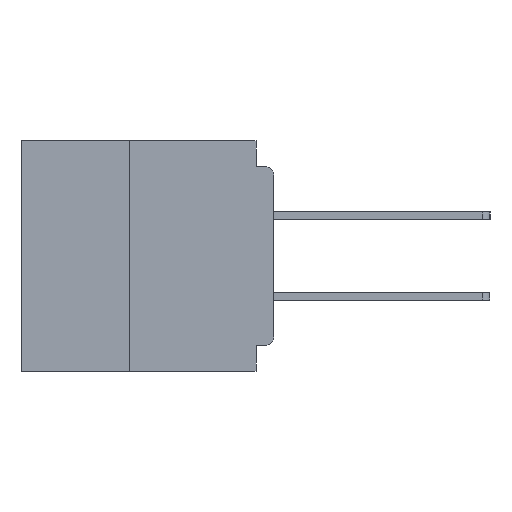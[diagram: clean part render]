
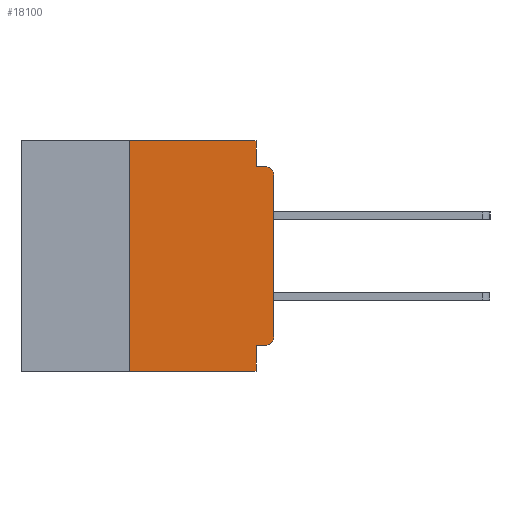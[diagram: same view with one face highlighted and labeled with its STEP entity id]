
A CAD part, left-side view. The second image highlights one B-rep face of the part: STEP entity #18100.
In plain terms, the highlighted planar face has unit normal (-1, 0, 0).
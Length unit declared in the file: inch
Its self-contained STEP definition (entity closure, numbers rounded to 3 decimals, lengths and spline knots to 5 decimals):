
#361 = VECTOR ( 'NONE', #4038, 39.37008 ) ;
#411 = CARTESIAN_POINT ( 'NONE',  ( 0., 0.031, -0.4 ) ) ;
#1312 = LINE ( 'NONE', #27914, #361 ) ;
#1744 = DIRECTION ( 'NONE',  ( 0., 0., -1. ) ) ;
#2793 = ORIENTED_EDGE ( 'NONE', *, *, #10416, .F. ) ;
#3578 = ORIENTED_EDGE ( 'NONE', *, *, #20698, .F. ) ;
#4038 = DIRECTION ( 'NONE',  ( 0., -1., 0. ) ) ;
#4580 = DIRECTION ( 'NONE',  ( 0., 1., 0. ) ) ;
#4935 = VECTOR ( 'NONE', #12124, 39.37008 ) ;
#5967 = VERTEX_POINT ( 'NONE', #23210 ) ;
#5987 = EDGE_CURVE ( 'NONE', #5967, #30522, #28568, .T. ) ;
#6387 = DIRECTION ( 'NONE',  ( 0., 0., -1. ) ) ;
#6660 = VECTOR ( 'NONE', #13336, 39.37008 ) ;
#6717 = EDGE_CURVE ( 'NONE', #25941, #8193, #11268, .T. ) ;
#6762 = VERTEX_POINT ( 'NONE', #13317 ) ;
#7190 = ORIENTED_EDGE ( 'NONE', *, *, #8110, .F. ) ;
#7269 = ORIENTED_EDGE ( 'NONE', *, *, #6717, .F. ) ;
#7526 = CIRCLE ( 'NONE', #22217, 0.015 ) ;
#7568 = LINE ( 'NONE', #28177, #6660 ) ;
#7718 = DIRECTION ( 'NONE',  ( -1., 0., 0. ) ) ;
#7893 = ORIENTED_EDGE ( 'NONE', *, *, #26180, .T. ) ;
#8110 = EDGE_CURVE ( 'NONE', #6762, #12100, #1312, .T. ) ;
#8193 = VERTEX_POINT ( 'NONE', #13462 ) ;
#8603 = EDGE_CURVE ( 'NONE', #12100, #25941, #36932, .T. ) ;
#9294 = FACE_OUTER_BOUND ( 'NONE', #30058, .T. ) ;
#10416 = EDGE_CURVE ( 'NONE', #21054, #30927, #36407, .T. ) ;
#10560 = CARTESIAN_POINT ( 'NONE',  ( 0., 0., -0.355 ) ) ;
#11268 = LINE ( 'NONE', #21096, #18243 ) ;
#11786 = VECTOR ( 'NONE', #23440, 39.37008 ) ;
#11883 = LINE ( 'NONE', #10560, #18884 ) ;
#12100 = VERTEX_POINT ( 'NONE', #33502 ) ;
#12124 = DIRECTION ( 'NONE',  ( 0., 0., -1. ) ) ;
#12818 = VECTOR ( 'NONE', #34408, 39.37008 ) ;
#13317 = CARTESIAN_POINT ( 'NONE',  ( 0., 0.25, 0. ) ) ;
#13336 = DIRECTION ( 'NONE',  ( 0., -1., 0. ) ) ;
#13462 = CARTESIAN_POINT ( 'NONE',  ( 0., 0.015, -0.045 ) ) ;
#13906 = DIRECTION ( 'NONE',  ( -1., 0., 0. ) ) ;
#14189 = DIRECTION ( 'NONE',  ( 0., -1., 0. ) ) ;
#15137 = CARTESIAN_POINT ( 'NONE',  ( 0., 0.031, -0.4 ) ) ;
#16322 = EDGE_CURVE ( 'NONE', #33196, #5967, #7526, .T. ) ;
#17006 = AXIS2_PLACEMENT_3D ( 'NONE', #37208, #19658, #1744 ) ;
#18100 = ADVANCED_FACE ( 'NONE', ( #9294 ), #34364, .F. ) ;
#18243 = VECTOR ( 'NONE', #14189, 39.37008 ) ;
#18400 = ORIENTED_EDGE ( 'NONE', *, *, #24849, .F. ) ;
#18544 = ORIENTED_EDGE ( 'NONE', *, *, #16322, .T. ) ;
#18545 = CIRCLE ( 'NONE', #19539, 0.015 ) ;
#18884 = VECTOR ( 'NONE', #4580, 39.37008 ) ;
#19513 = CARTESIAN_POINT ( 'NONE',  ( 0., 0., -0.06 ) ) ;
#19539 = AXIS2_PLACEMENT_3D ( 'NONE', #25599, #7718, #28581 ) ;
#19658 = DIRECTION ( 'NONE',  ( 1., 0., 0. ) ) ;
#20698 = EDGE_CURVE ( 'NONE', #33196, #21054, #11883, .T. ) ;
#21054 = VERTEX_POINT ( 'NONE', #21104 ) ;
#21096 = CARTESIAN_POINT ( 'NONE',  ( 0., 0., -0.045 ) ) ;
#21104 = CARTESIAN_POINT ( 'NONE',  ( 0., 0.031, -0.355 ) ) ;
#21702 = VERTEX_POINT ( 'NONE', #35594 ) ;
#22217 = AXIS2_PLACEMENT_3D ( 'NONE', #31675, #13906, #34592 ) ;
#23210 = CARTESIAN_POINT ( 'NONE',  ( 0., 0., -0.34 ) ) ;
#23440 = DIRECTION ( 'NONE',  ( 0., 0., 1. ) ) ;
#23975 = CARTESIAN_POINT ( 'NONE',  ( 0., 0., 0. ) ) ;
#24038 = CARTESIAN_POINT ( 'NONE',  ( 0., 0.031, -0.045 ) ) ;
#24849 = EDGE_CURVE ( 'NONE', #21702, #6762, #36338, .T. ) ;
#25599 = CARTESIAN_POINT ( 'NONE',  ( 0., 0.015, -0.06 ) ) ;
#25941 = VERTEX_POINT ( 'NONE', #24038 ) ;
#26180 = EDGE_CURVE ( 'NONE', #21702, #30927, #7568, .T. ) ;
#27286 = ORIENTED_EDGE ( 'NONE', *, *, #8603, .F. ) ;
#27914 = CARTESIAN_POINT ( 'NONE',  ( 0., 0.437, 0. ) ) ;
#28177 = CARTESIAN_POINT ( 'NONE',  ( 0., 0.437, -0.4 ) ) ;
#28568 = LINE ( 'NONE', #23975, #11786 ) ;
#28581 = DIRECTION ( 'NONE',  ( 0., 0., -1. ) ) ;
#29275 = VECTOR ( 'NONE', #6387, 39.37008 ) ;
#29369 = ORIENTED_EDGE ( 'NONE', *, *, #5987, .T. ) ;
#30058 = EDGE_LOOP ( 'NONE', ( #29369, #33307, #7269, #27286, #7190, #18400, #7893, #2793, #3578, #18544 ) ) ;
#30522 = VERTEX_POINT ( 'NONE', #19513 ) ;
#30927 = VERTEX_POINT ( 'NONE', #411 ) ;
#31485 = CARTESIAN_POINT ( 'NONE',  ( 0., 0.25, -0.4 ) ) ;
#31675 = CARTESIAN_POINT ( 'NONE',  ( 0., 0.015, -0.34 ) ) ;
#33196 = VERTEX_POINT ( 'NONE', #34727 ) ;
#33307 = ORIENTED_EDGE ( 'NONE', *, *, #34625, .T. ) ;
#33502 = CARTESIAN_POINT ( 'NONE',  ( 0., 0.031, 0. ) ) ;
#34364 = PLANE ( 'NONE',  #17006 ) ;
#34408 = DIRECTION ( 'NONE',  ( 0., 0., 1. ) ) ;
#34592 = DIRECTION ( 'NONE',  ( 0., 0., -1. ) ) ;
#34625 = EDGE_CURVE ( 'NONE', #30522, #8193, #18545, .T. ) ;
#34727 = CARTESIAN_POINT ( 'NONE',  ( 0., 0.015, -0.355 ) ) ;
#35594 = CARTESIAN_POINT ( 'NONE',  ( 0., 0.25, -0.4 ) ) ;
#35890 = CARTESIAN_POINT ( 'NONE',  ( 0., 0.031, 0. ) ) ;
#36338 = LINE ( 'NONE', #31485, #12818 ) ;
#36407 = LINE ( 'NONE', #15137, #4935 ) ;
#36932 = LINE ( 'NONE', #35890, #29275 ) ;
#37208 = CARTESIAN_POINT ( 'NONE',  ( 0., 0.437, 0. ) ) ;
